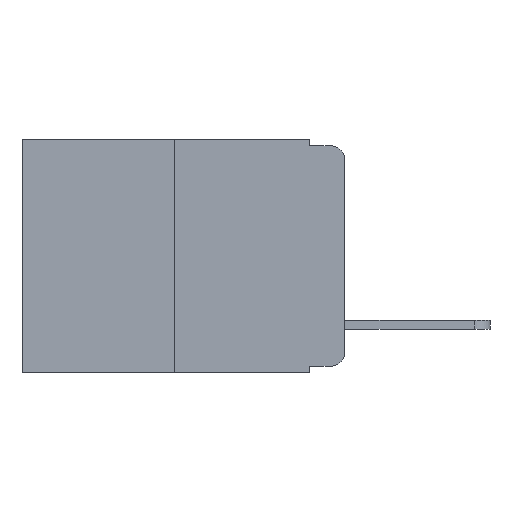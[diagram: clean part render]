
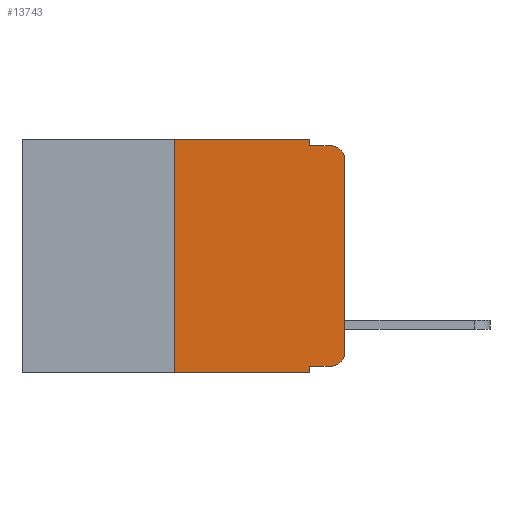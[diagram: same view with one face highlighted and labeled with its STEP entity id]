
A CAD part, left-side view. The second image highlights one B-rep face of the part: STEP entity #13743.
In plain terms, the highlighted planar face has unit normal (-1, 0, 0).
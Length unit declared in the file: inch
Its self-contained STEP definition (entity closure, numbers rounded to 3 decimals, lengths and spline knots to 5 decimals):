
#210 = LINE ( 'NONE', #13632, #5269 ) ;
#498 = ORIENTED_EDGE ( 'NONE', *, *, #1928, .F. ) ;
#765 = FACE_OUTER_BOUND ( 'NONE', #7772, .T. ) ;
#971 = EDGE_CURVE ( 'NONE', #12981, #3849, #8546, .T. ) ;
#1928 = EDGE_CURVE ( 'NONE', #13045, #17584, #210, .T. ) ;
#2074 = EDGE_CURVE ( 'NONE', #10723, #7954, #16825, .T. ) ;
#2270 = ORIENTED_EDGE ( 'NONE', *, *, #8079, .F. ) ;
#2606 = LINE ( 'NONE', #21629, #22808 ) ;
#2778 = ORIENTED_EDGE ( 'NONE', *, *, #22235, .F. ) ;
#3033 = ORIENTED_EDGE ( 'NONE', *, *, #14577, .T. ) ;
#3116 = VECTOR ( 'NONE', #3973, 39.37008 ) ;
#3273 = CARTESIAN_POINT ( 'NONE',  ( 0., 0.25, 0. ) ) ;
#3355 = VERTEX_POINT ( 'NONE', #23702 ) ;
#3849 = VERTEX_POINT ( 'NONE', #10918 ) ;
#3973 = DIRECTION ( 'NONE',  ( 0., 0., 1. ) ) ;
#4058 = PLANE ( 'NONE',  #15353 ) ;
#4310 = VECTOR ( 'NONE', #11502, 39.37008 ) ;
#4362 = DIRECTION ( 'NONE',  ( 0., -1., 0. ) ) ;
#4425 = CARTESIAN_POINT ( 'NONE',  ( 0., 0.051, -0.333 ) ) ;
#4469 = ORIENTED_EDGE ( 'NONE', *, *, #2074, .F. ) ;
#4556 = ORIENTED_EDGE ( 'NONE', *, *, #6897, .T. ) ;
#4875 = VECTOR ( 'NONE', #12925, 39.37008 ) ;
#5269 = VECTOR ( 'NONE', #5886, 39.37008 ) ;
#5625 = VERTEX_POINT ( 'NONE', #10704 ) ;
#5851 = VECTOR ( 'NONE', #21012, 39.37008 ) ;
#5886 = DIRECTION ( 'NONE',  ( 0., -1., 0. ) ) ;
#6015 = DIRECTION ( 'NONE',  ( 0., -1., 0. ) ) ;
#6116 = DIRECTION ( 'NONE',  ( 1., 0., 0. ) ) ;
#6704 = EDGE_CURVE ( 'NONE', #12981, #15414, #7186, .T. ) ;
#6897 = EDGE_CURVE ( 'NONE', #13432, #15414, #2606, .T. ) ;
#6958 = DIRECTION ( 'NONE',  ( -1., 0., 0. ) ) ;
#7186 = LINE ( 'NONE', #22709, #4310 ) ;
#7772 = EDGE_LOOP ( 'NONE', ( #24698, #8062, #498, #2778, #4469, #2270, #4556, #11108, #22789, #3033 ) ) ;
#7892 = VECTOR ( 'NONE', #4362, 39.37008 ) ;
#7954 = VERTEX_POINT ( 'NONE', #13024 ) ;
#7998 = CARTESIAN_POINT ( 'NONE',  ( 0., 0., 0. ) ) ;
#8062 = ORIENTED_EDGE ( 'NONE', *, *, #10320, .T. ) ;
#8079 = EDGE_CURVE ( 'NONE', #13432, #10723, #16505, .T. ) ;
#8521 = CARTESIAN_POINT ( 'NONE',  ( 0., 0.25, 0. ) ) ;
#8546 = LINE ( 'NONE', #24752, #7892 ) ;
#8889 = CARTESIAN_POINT ( 'NONE',  ( 0., 0.051, 0. ) ) ;
#9004 = DIRECTION ( 'NONE',  ( -1., 0., 0. ) ) ;
#10320 = EDGE_CURVE ( 'NONE', #3355, #17584, #18398, .T. ) ;
#10703 = CARTESIAN_POINT ( 'NONE',  ( 0., 0.473, 0. ) ) ;
#10704 = CARTESIAN_POINT ( 'NONE',  ( 0., 0., -0.313 ) ) ;
#10723 = VERTEX_POINT ( 'NONE', #8521 ) ;
#10918 = CARTESIAN_POINT ( 'NONE',  ( 0., 0.02, -0.333 ) ) ;
#11108 = ORIENTED_EDGE ( 'NONE', *, *, #6704, .F. ) ;
#11502 = DIRECTION ( 'NONE',  ( 0., 0., -1. ) ) ;
#11704 = VECTOR ( 'NONE', #6015, 39.37008 ) ;
#12925 = DIRECTION ( 'NONE',  ( 0., 0., -1. ) ) ;
#12981 = VERTEX_POINT ( 'NONE', #4425 ) ;
#13024 = CARTESIAN_POINT ( 'NONE',  ( 0., 0.051, 0. ) ) ;
#13045 = VERTEX_POINT ( 'NONE', #22185 ) ;
#13432 = VERTEX_POINT ( 'NONE', #23503 ) ;
#13632 = CARTESIAN_POINT ( 'NONE',  ( 0., 0.051, -0.01 ) ) ;
#13743 = ADVANCED_FACE ( 'NONE', ( #765 ), #4058, .F. ) ;
#14160 = CARTESIAN_POINT ( 'NONE',  ( 0., 0.473, 0. ) ) ;
#14577 = EDGE_CURVE ( 'NONE', #3849, #5625, #24942, .T. ) ;
#15353 = AXIS2_PLACEMENT_3D ( 'NONE', #14160, #6116, #19835 ) ;
#15414 = VERTEX_POINT ( 'NONE', #17260 ) ;
#15663 = EDGE_CURVE ( 'NONE', #5625, #3355, #23220, .T. ) ;
#16505 = LINE ( 'NONE', #3273, #5851 ) ;
#16825 = LINE ( 'NONE', #10703, #11704 ) ;
#17260 = CARTESIAN_POINT ( 'NONE',  ( 0., 0.051, -0.343 ) ) ;
#17584 = VERTEX_POINT ( 'NONE', #22218 ) ;
#17943 = DIRECTION ( 'NONE',  ( 0., -1., 0. ) ) ;
#18398 = CIRCLE ( 'NONE', #21884, 0.02 ) ;
#18751 = CARTESIAN_POINT ( 'NONE',  ( 0., 0.02, -0.313 ) ) ;
#19835 = DIRECTION ( 'NONE',  ( 0., 0., -1. ) ) ;
#20551 = CARTESIAN_POINT ( 'NONE',  ( 0., 0.02, -0.03 ) ) ;
#20592 = DIRECTION ( 'NONE',  ( 0., 0., -1. ) ) ;
#21012 = DIRECTION ( 'NONE',  ( 0., 0., 1. ) ) ;
#21629 = CARTESIAN_POINT ( 'NONE',  ( 0., 0.473, -0.343 ) ) ;
#21884 = AXIS2_PLACEMENT_3D ( 'NONE', #20551, #9004, #22340 ) ;
#22185 = CARTESIAN_POINT ( 'NONE',  ( 0., 0.051, -0.01 ) ) ;
#22218 = CARTESIAN_POINT ( 'NONE',  ( 0., 0.02, -0.01 ) ) ;
#22235 = EDGE_CURVE ( 'NONE', #7954, #13045, #25259, .T. ) ;
#22340 = DIRECTION ( 'NONE',  ( 0., 0., -1. ) ) ;
#22550 = AXIS2_PLACEMENT_3D ( 'NONE', #18751, #6958, #20592 ) ;
#22709 = CARTESIAN_POINT ( 'NONE',  ( 0., 0.051, 0. ) ) ;
#22789 = ORIENTED_EDGE ( 'NONE', *, *, #971, .T. ) ;
#22808 = VECTOR ( 'NONE', #17943, 39.37008 ) ;
#23220 = LINE ( 'NONE', #7998, #3116 ) ;
#23503 = CARTESIAN_POINT ( 'NONE',  ( 0., 0.25, -0.343 ) ) ;
#23702 = CARTESIAN_POINT ( 'NONE',  ( 0., 0., -0.03 ) ) ;
#24698 = ORIENTED_EDGE ( 'NONE', *, *, #15663, .T. ) ;
#24752 = CARTESIAN_POINT ( 'NONE',  ( 0., 0.051, -0.333 ) ) ;
#24942 = CIRCLE ( 'NONE', #22550, 0.02 ) ;
#25259 = LINE ( 'NONE', #8889, #4875 ) ;
